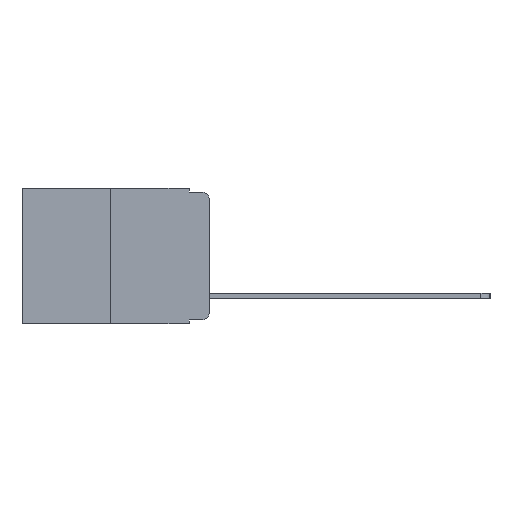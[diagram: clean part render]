
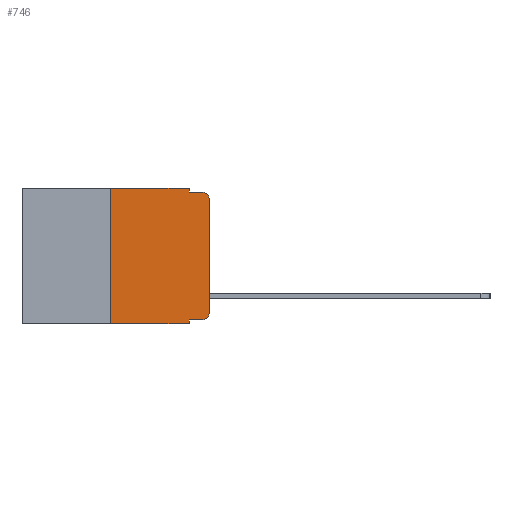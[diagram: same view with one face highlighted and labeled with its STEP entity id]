
A CAD part, left-side view. The second image highlights one B-rep face of the part: STEP entity #746.
In plain terms, the highlighted planar face has unit normal (-1, 0, 0).
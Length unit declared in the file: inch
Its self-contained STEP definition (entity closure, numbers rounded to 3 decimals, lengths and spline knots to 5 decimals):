
#447 = CARTESIAN_POINT ( 'NONE',  ( 0., 0.051, -0.333 ) ) ;
#746 = ADVANCED_FACE ( 'NONE', ( #11334 ), #9230, .F. ) ;
#1074 = EDGE_CURVE ( 'NONE', #3684, #9562, #6449, .T. ) ;
#1130 = CARTESIAN_POINT ( 'NONE',  ( 0., 0.25, 0. ) ) ;
#1351 = CIRCLE ( 'NONE', #10835, 0.02 ) ;
#1569 = VERTEX_POINT ( 'NONE', #7511 ) ;
#1744 = CARTESIAN_POINT ( 'NONE',  ( 0., 0.02, -0.333 ) ) ;
#1762 = VECTOR ( 'NONE', #11183, 39.37008 ) ;
#2129 = DIRECTION ( 'NONE',  ( 0., 0., -1. ) ) ;
#2154 = EDGE_CURVE ( 'NONE', #4060, #6536, #11976, .T. ) ;
#2518 = EDGE_CURVE ( 'NONE', #11652, #9519, #3999, .T. ) ;
#2538 = ORIENTED_EDGE ( 'NONE', *, *, #2584, .T. ) ;
#2584 = EDGE_CURVE ( 'NONE', #12956, #11652, #5831, .T. ) ;
#2600 = EDGE_CURVE ( 'NONE', #12956, #9562, #12829, .T. ) ;
#2630 = EDGE_CURVE ( 'NONE', #3684, #4060, #12542, .T. ) ;
#2650 = EDGE_CURVE ( 'NONE', #6536, #5461, #7394, .T. ) ;
#2651 = EDGE_CURVE ( 'NONE', #5461, #8687, #10147, .T. ) ;
#2657 = ORIENTED_EDGE ( 'NONE', *, *, #2651, .F. ) ;
#2675 = EDGE_CURVE ( 'NONE', #1569, #8687, #1351, .T. ) ;
#2689 = EDGE_CURVE ( 'NONE', #9519, #1569, #11679, .T. ) ;
#2743 = DIRECTION ( 'NONE',  ( 1., 0., 0. ) ) ;
#3001 = DIRECTION ( 'NONE',  ( 0., 0., 1. ) ) ;
#3029 = CARTESIAN_POINT ( 'NONE',  ( 0., 0.051, -0.343 ) ) ;
#3042 = DIRECTION ( 'NONE',  ( 0., 0., -1. ) ) ;
#3121 = CARTESIAN_POINT ( 'NONE',  ( 0., 0.051, 0. ) ) ;
#3221 = ORIENTED_EDGE ( 'NONE', *, *, #2689, .T. ) ;
#3438 = ORIENTED_EDGE ( 'NONE', *, *, #2154, .F. ) ;
#3618 = CARTESIAN_POINT ( 'NONE',  ( 0., 0.25, -0.343 ) ) ;
#3684 = VERTEX_POINT ( 'NONE', #3618 ) ;
#3825 = VECTOR ( 'NONE', #3001, 39.37008 ) ;
#3999 = CIRCLE ( 'NONE', #5604, 0.02 ) ;
#4060 = VERTEX_POINT ( 'NONE', #1130 ) ;
#4205 = AXIS2_PLACEMENT_3D ( 'NONE', #5198, #2743, #2129 ) ;
#4491 = VECTOR ( 'NONE', #12533, 39.37008 ) ;
#4522 = VECTOR ( 'NONE', #7615, 39.37008 ) ;
#4663 = ORIENTED_EDGE ( 'NONE', *, *, #2630, .F. ) ;
#4761 = DIRECTION ( 'NONE',  ( 0., 0., -1. ) ) ;
#4790 = DIRECTION ( 'NONE',  ( -1., 0., 0. ) ) ;
#4805 = CARTESIAN_POINT ( 'NONE',  ( 0., 0.02, -0.313 ) ) ;
#4845 = VECTOR ( 'NONE', #10821, 39.37008 ) ;
#4902 = CARTESIAN_POINT ( 'NONE',  ( 0., 0.051, 0. ) ) ;
#4952 = ORIENTED_EDGE ( 'NONE', *, *, #1074, .T. ) ;
#5073 = CARTESIAN_POINT ( 'NONE',  ( 0., 0.051, -0.01 ) ) ;
#5198 = CARTESIAN_POINT ( 'NONE',  ( 0., 0.473, 0. ) ) ;
#5461 = VERTEX_POINT ( 'NONE', #5073 ) ;
#5503 = VECTOR ( 'NONE', #12439, 39.37008 ) ;
#5604 = AXIS2_PLACEMENT_3D ( 'NONE', #4805, #4790, #4761 ) ;
#5831 = LINE ( 'NONE', #447, #5503 ) ;
#6449 = LINE ( 'NONE', #11132, #11178 ) ;
#6536 = VERTEX_POINT ( 'NONE', #13037 ) ;
#6733 = EDGE_LOOP ( 'NONE', ( #3221, #8289, #2657, #8539, #3438, #4663, #4952, #9601, #2538, #8742 ) ) ;
#7356 = DIRECTION ( 'NONE',  ( 0., 0., -1. ) ) ;
#7394 = LINE ( 'NONE', #4902, #4491 ) ;
#7511 = CARTESIAN_POINT ( 'NONE',  ( 0., 0., -0.03 ) ) ;
#7545 = CARTESIAN_POINT ( 'NONE',  ( 0., 0.02, -0.01 ) ) ;
#7615 = DIRECTION ( 'NONE',  ( 0., -1., 0. ) ) ;
#8282 = VECTOR ( 'NONE', #3042, 39.37008 ) ;
#8289 = ORIENTED_EDGE ( 'NONE', *, *, #2675, .T. ) ;
#8302 = CARTESIAN_POINT ( 'NONE',  ( 0., 0., -0.313 ) ) ;
#8539 = ORIENTED_EDGE ( 'NONE', *, *, #2650, .F. ) ;
#8687 = VERTEX_POINT ( 'NONE', #7545 ) ;
#8742 = ORIENTED_EDGE ( 'NONE', *, *, #2518, .T. ) ;
#9230 = PLANE ( 'NONE',  #4205 ) ;
#9519 = VERTEX_POINT ( 'NONE', #8302 ) ;
#9562 = VERTEX_POINT ( 'NONE', #3029 ) ;
#9601 = ORIENTED_EDGE ( 'NONE', *, *, #2600, .F. ) ;
#10059 = CARTESIAN_POINT ( 'NONE',  ( 0., 0.051, -0.01 ) ) ;
#10147 = LINE ( 'NONE', #10059, #1762 ) ;
#10437 = CARTESIAN_POINT ( 'NONE',  ( 0., 0.051, -0.333 ) ) ;
#10821 = DIRECTION ( 'NONE',  ( 0., 0., 1. ) ) ;
#10835 = AXIS2_PLACEMENT_3D ( 'NONE', #13096, #12218, #7356 ) ;
#11132 = CARTESIAN_POINT ( 'NONE',  ( 0., 0.473, -0.343 ) ) ;
#11178 = VECTOR ( 'NONE', #12467, 39.37008 ) ;
#11183 = DIRECTION ( 'NONE',  ( 0., -1., 0. ) ) ;
#11334 = FACE_OUTER_BOUND ( 'NONE', #6733, .T. ) ;
#11652 = VERTEX_POINT ( 'NONE', #1744 ) ;
#11679 = LINE ( 'NONE', #13483, #3825 ) ;
#11876 = CARTESIAN_POINT ( 'NONE',  ( 0., 0.25, 0. ) ) ;
#11976 = LINE ( 'NONE', #12275, #4522 ) ;
#12218 = DIRECTION ( 'NONE',  ( -1., 0., 0. ) ) ;
#12275 = CARTESIAN_POINT ( 'NONE',  ( 0., 0.473, 0. ) ) ;
#12439 = DIRECTION ( 'NONE',  ( 0., -1., 0. ) ) ;
#12467 = DIRECTION ( 'NONE',  ( 0., -1., 0. ) ) ;
#12533 = DIRECTION ( 'NONE',  ( 0., 0., -1. ) ) ;
#12542 = LINE ( 'NONE', #11876, #4845 ) ;
#12829 = LINE ( 'NONE', #3121, #8282 ) ;
#12956 = VERTEX_POINT ( 'NONE', #10437 ) ;
#13037 = CARTESIAN_POINT ( 'NONE',  ( 0., 0.051, 0. ) ) ;
#13096 = CARTESIAN_POINT ( 'NONE',  ( 0., 0.02, -0.03 ) ) ;
#13483 = CARTESIAN_POINT ( 'NONE',  ( 0., 0., 0. ) ) ;
